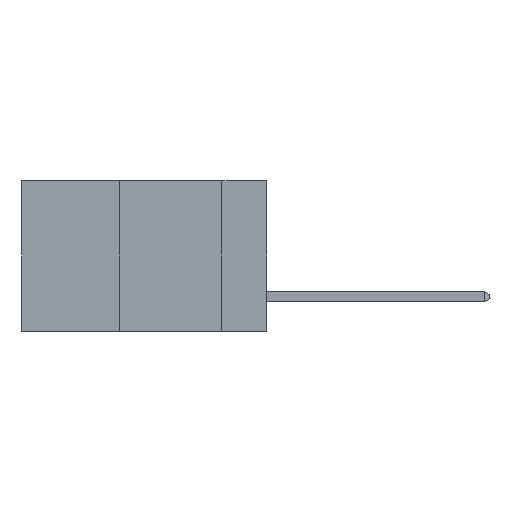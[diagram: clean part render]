
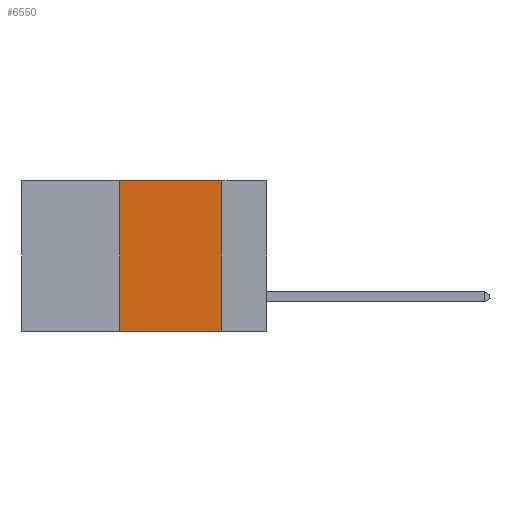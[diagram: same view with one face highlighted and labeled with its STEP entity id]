
A CAD part, left-side view. The second image highlights one B-rep face of the part: STEP entity #6550.
In plain terms, the highlighted planar face has unit normal (-1, 0, 0).
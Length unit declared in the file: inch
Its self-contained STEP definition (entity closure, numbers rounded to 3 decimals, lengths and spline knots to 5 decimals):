
#297 = EDGE_CURVE ( 'NONE', #13258, #17195, #14675, .T. ) ;
#845 = ORIENTED_EDGE ( 'NONE', *, *, #297, .F. ) ;
#939 = DIRECTION ( 'NONE',  ( 0., -1., 0. ) ) ;
#1072 = PLANE ( 'NONE',  #11072 ) ;
#2106 = CARTESIAN_POINT ( 'NONE',  ( 0., 0.36, 0. ) ) ;
#2354 = CARTESIAN_POINT ( 'NONE',  ( 0., 0.6, 0. ) ) ;
#2831 = DIRECTION ( 'NONE',  ( 0., 0., -1. ) ) ;
#3924 = ORIENTED_EDGE ( 'NONE', *, *, #17822, .F. ) ;
#4128 = VERTEX_POINT ( 'NONE', #6655 ) ;
#4399 = ORIENTED_EDGE ( 'NONE', *, *, #6612, .T. ) ;
#4609 = CARTESIAN_POINT ( 'NONE',  ( 0., 0.36, 0. ) ) ;
#5061 = CARTESIAN_POINT ( 'NONE',  ( 0., 0.6, 0. ) ) ;
#5867 = LINE ( 'NONE', #5061, #13157 ) ;
#5972 = FACE_OUTER_BOUND ( 'NONE', #18665, .T. ) ;
#6071 = VERTEX_POINT ( 'NONE', #15907 ) ;
#6370 = LINE ( 'NONE', #8987, #7846 ) ;
#6550 = ADVANCED_FACE ( 'NONE', ( #5972 ), #1072, .F. ) ;
#6612 = EDGE_CURVE ( 'NONE', #13258, #6071, #10005, .T. ) ;
#6655 = CARTESIAN_POINT ( 'NONE',  ( 0., 0.11, 0. ) ) ;
#7472 = VECTOR ( 'NONE', #19338, 39.37008 ) ;
#7846 = VECTOR ( 'NONE', #2831, 39.37008 ) ;
#8987 = CARTESIAN_POINT ( 'NONE',  ( 0., 0.11, 0. ) ) ;
#10005 = LINE ( 'NONE', #18911, #13755 ) ;
#10041 = DIRECTION ( 'NONE',  ( 0., -1., 0. ) ) ;
#11072 = AXIS2_PLACEMENT_3D ( 'NONE', #2354, #11410, #14624 ) ;
#11410 = DIRECTION ( 'NONE',  ( 1., 0., 0. ) ) ;
#12704 = CARTESIAN_POINT ( 'NONE',  ( 0., 0.36, -0.37 ) ) ;
#13157 = VECTOR ( 'NONE', #939, 39.37008 ) ;
#13258 = VERTEX_POINT ( 'NONE', #12704 ) ;
#13755 = VECTOR ( 'NONE', #10041, 39.37008 ) ;
#14624 = DIRECTION ( 'NONE',  ( 0., 0., -1. ) ) ;
#14675 = LINE ( 'NONE', #4609, #7472 ) ;
#15907 = CARTESIAN_POINT ( 'NONE',  ( 0., 0.11, -0.37 ) ) ;
#17195 = VERTEX_POINT ( 'NONE', #2106 ) ;
#17317 = ORIENTED_EDGE ( 'NONE', *, *, #17510, .F. ) ;
#17510 = EDGE_CURVE ( 'NONE', #4128, #6071, #6370, .T. ) ;
#17822 = EDGE_CURVE ( 'NONE', #17195, #4128, #5867, .T. ) ;
#18665 = EDGE_LOOP ( 'NONE', ( #17317, #3924, #845, #4399 ) ) ;
#18911 = CARTESIAN_POINT ( 'NONE',  ( 0., 0.6, -0.37 ) ) ;
#19338 = DIRECTION ( 'NONE',  ( 0., 0., 1. ) ) ;
